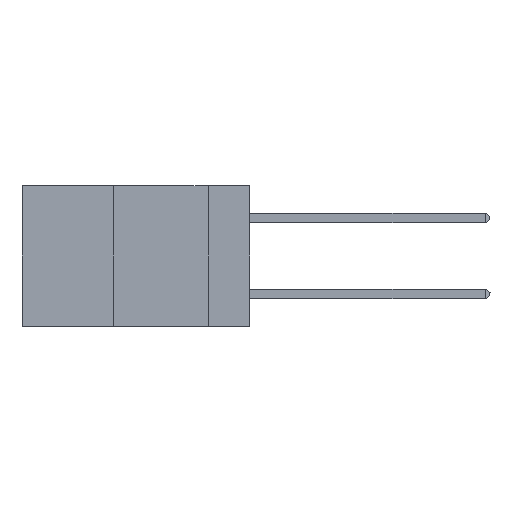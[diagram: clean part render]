
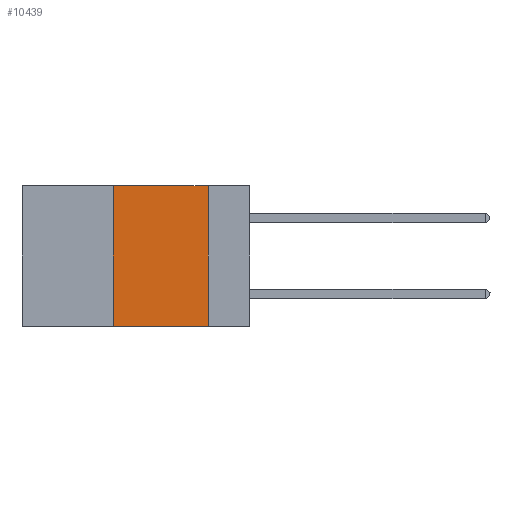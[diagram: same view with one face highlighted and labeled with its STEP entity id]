
A CAD part, left-side view. The second image highlights one B-rep face of the part: STEP entity #10439.
In plain terms, the highlighted planar face has unit normal (-1, 0, 0).
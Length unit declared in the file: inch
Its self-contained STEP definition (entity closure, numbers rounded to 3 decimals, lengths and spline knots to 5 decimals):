
#1255 = DIRECTION ( 'NONE',  ( 0., 0., -1. ) ) ;
#1361 = CARTESIAN_POINT ( 'NONE',  ( 0., 0.11, 0. ) ) ;
#2413 = LINE ( 'NONE', #23666, #26877 ) ;
#3650 = VERTEX_POINT ( 'NONE', #13528 ) ;
#4030 = EDGE_CURVE ( 'NONE', #17018, #3650, #2413, .T. ) ;
#5005 = LINE ( 'NONE', #7092, #22640 ) ;
#5733 = VERTEX_POINT ( 'NONE', #26355 ) ;
#7092 = CARTESIAN_POINT ( 'NONE',  ( 0., 0.6, -0.37 ) ) ;
#8802 = PLANE ( 'NONE',  #24088 ) ;
#9356 = CARTESIAN_POINT ( 'NONE',  ( 0., 0.36, -0.37 ) ) ;
#9507 = DIRECTION ( 'NONE',  ( 0., 0., 1. ) ) ;
#9571 = ORIENTED_EDGE ( 'NONE', *, *, #4030, .F. ) ;
#9627 = LINE ( 'NONE', #25028, #17559 ) ;
#10439 = ADVANCED_FACE ( 'NONE', ( #20933 ), #8802, .F. ) ;
#11671 = ORIENTED_EDGE ( 'NONE', *, *, #25815, .F. ) ;
#11966 = EDGE_CURVE ( 'NONE', #13918, #5733, #5005, .T. ) ;
#13410 = EDGE_CURVE ( 'NONE', #13918, #17018, #9627, .T. ) ;
#13528 = CARTESIAN_POINT ( 'NONE',  ( 0., 0.11, 0. ) ) ;
#13918 = VERTEX_POINT ( 'NONE', #9356 ) ;
#14045 = CARTESIAN_POINT ( 'NONE',  ( 0., 0.36, 0. ) ) ;
#15379 = DIRECTION ( 'NONE',  ( 0., 0., -1. ) ) ;
#17018 = VERTEX_POINT ( 'NONE', #14045 ) ;
#17559 = VECTOR ( 'NONE', #9507, 39.37008 ) ;
#19408 = LINE ( 'NONE', #1361, #23737 ) ;
#20933 = FACE_OUTER_BOUND ( 'NONE', #22924, .T. ) ;
#21272 = ORIENTED_EDGE ( 'NONE', *, *, #13410, .F. ) ;
#22640 = VECTOR ( 'NONE', #26005, 39.37008 ) ;
#22924 = EDGE_LOOP ( 'NONE', ( #11671, #9571, #21272, #28795 ) ) ;
#23666 = CARTESIAN_POINT ( 'NONE',  ( 0., 0.6, 0. ) ) ;
#23737 = VECTOR ( 'NONE', #1255, 39.37008 ) ;
#24088 = AXIS2_PLACEMENT_3D ( 'NONE', #29526, #27128, #15379 ) ;
#25028 = CARTESIAN_POINT ( 'NONE',  ( 0., 0.36, 0. ) ) ;
#25815 = EDGE_CURVE ( 'NONE', #3650, #5733, #19408, .T. ) ;
#26005 = DIRECTION ( 'NONE',  ( 0., -1., 0. ) ) ;
#26355 = CARTESIAN_POINT ( 'NONE',  ( 0., 0.11, -0.37 ) ) ;
#26877 = VECTOR ( 'NONE', #28697, 39.37008 ) ;
#27128 = DIRECTION ( 'NONE',  ( 1., 0., 0. ) ) ;
#28697 = DIRECTION ( 'NONE',  ( 0., -1., 0. ) ) ;
#28795 = ORIENTED_EDGE ( 'NONE', *, *, #11966, .T. ) ;
#29526 = CARTESIAN_POINT ( 'NONE',  ( 0., 0.6, 0. ) ) ;
